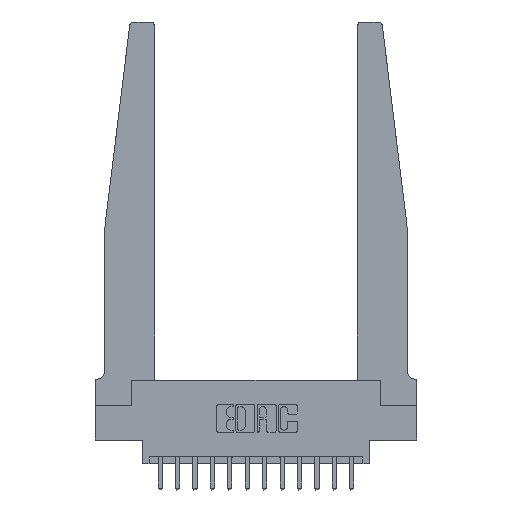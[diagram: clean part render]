
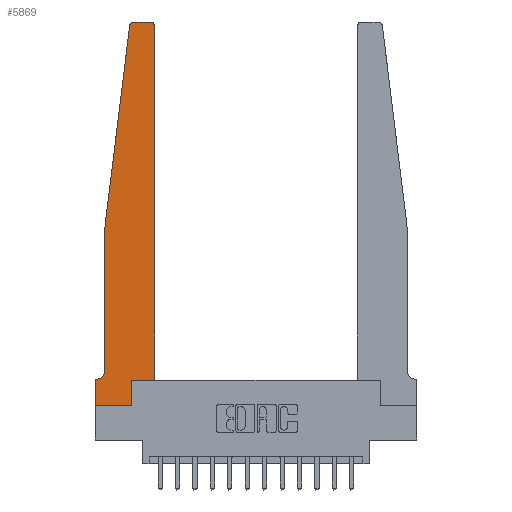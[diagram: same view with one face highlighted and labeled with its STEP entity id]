
A CAD part, top view. The second image highlights one B-rep face of the part: STEP entity #5869.
In plain terms, the highlighted planar face has unit normal (0, 0, 1).
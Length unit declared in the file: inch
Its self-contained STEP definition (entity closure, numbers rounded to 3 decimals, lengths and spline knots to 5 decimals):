
#121 = ORIENTED_EDGE ( 'NONE', *, *, #11067, .T. ) ;
#284 = LINE ( 'NONE', #6180, #6841 ) ;
#321 = EDGE_CURVE ( 'NONE', #11823, #12574, #5708, .T. ) ;
#346 = DIRECTION ( 'NONE',  ( 1., 0., 0. ) ) ;
#353 = CARTESIAN_POINT ( 'NONE',  ( 0.065, 0.2375, 0.37 ) ) ;
#361 = CARTESIAN_POINT ( 'NONE',  ( 0., 0., 0.37 ) ) ;
#403 = CIRCLE ( 'NONE', #14187, 0.05 ) ;
#616 = VECTOR ( 'NONE', #904, 39.37008 ) ;
#721 = CARTESIAN_POINT ( 'NONE',  ( 0.015, 0.1875, 0.37 ) ) ;
#904 = DIRECTION ( 'NONE',  ( -1., 0., 0. ) ) ;
#1146 = DIRECTION ( 'NONE',  ( 0., -1., 0. ) ) ;
#1235 = CARTESIAN_POINT ( 'NONE',  ( 0.065, 1.25, 0.37 ) ) ;
#1589 = VERTEX_POINT ( 'NONE', #13075 ) ;
#1968 = VERTEX_POINT ( 'NONE', #13344 ) ;
#2219 = DIRECTION ( 'NONE',  ( 0., -1., 0. ) ) ;
#2501 = VECTOR ( 'NONE', #2949, 39.37008 ) ;
#2730 = VERTEX_POINT ( 'NONE', #353 ) ;
#2949 = DIRECTION ( 'NONE',  ( 0., 1., 0. ) ) ;
#2978 = LINE ( 'NONE', #1235, #16077 ) ;
#3011 = DIRECTION ( 'NONE',  ( 0., 0., -1. ) ) ;
#3089 = VECTOR ( 'NONE', #10060, 39.37008 ) ;
#3243 = ORIENTED_EDGE ( 'NONE', *, *, #4909, .T. ) ;
#3273 = EDGE_CURVE ( 'NONE', #12574, #16125, #6005, .T. ) ;
#3669 = LINE ( 'NONE', #13989, #616 ) ;
#3678 = CARTESIAN_POINT ( 'NONE',  ( 0.425, 0.18, 0.37 ) ) ;
#3949 = CARTESIAN_POINT ( 'NONE',  ( 0.2605, 0.18, 0.37 ) ) ;
#4288 = CARTESIAN_POINT ( 'NONE',  ( 0., 0.1875, 0.37 ) ) ;
#4425 = LINE ( 'NONE', #361, #4828 ) ;
#4828 = VECTOR ( 'NONE', #346, 39.37008 ) ;
#4901 = CIRCLE ( 'NONE', #8068, 0.03 ) ;
#4909 = EDGE_CURVE ( 'NONE', #10170, #2730, #2978, .T. ) ;
#4979 = CARTESIAN_POINT ( 'NONE',  ( 0.2605, 0.18, 0.37 ) ) ;
#5010 = EDGE_CURVE ( 'NONE', #1589, #12169, #4425, .T. ) ;
#5607 = DIRECTION ( 'NONE',  ( -1., 0., 0. ) ) ;
#5708 = LINE ( 'NONE', #9961, #8782 ) ;
#5761 = ORIENTED_EDGE ( 'NONE', *, *, #14147, .T. ) ;
#5869 = ADVANCED_FACE ( 'NONE', ( #16039 ), #11038, .T. ) ;
#5929 = CARTESIAN_POINT ( 'NONE',  ( 0.065, 1.25, 0.37 ) ) ;
#6005 = LINE ( 'NONE', #3678, #2501 ) ;
#6180 = CARTESIAN_POINT ( 'NONE',  ( 0., 0., 0.37 ) ) ;
#6351 = DIRECTION ( 'NONE',  ( 0., 0., 1. ) ) ;
#6604 = ORIENTED_EDGE ( 'NONE', *, *, #5010, .T. ) ;
#6641 = DIRECTION ( 'NONE',  ( 0., 0., 1. ) ) ;
#6841 = VECTOR ( 'NONE', #2219, 39.37008 ) ;
#7129 = LINE ( 'NONE', #3949, #13311 ) ;
#7538 = EDGE_CURVE ( 'NONE', #1968, #10170, #10120, .T. ) ;
#8068 = AXIS2_PLACEMENT_3D ( 'NONE', #14211, #6351, #15494 ) ;
#8175 = DIRECTION ( 'NONE',  ( 1., 0., 0. ) ) ;
#8308 = CARTESIAN_POINT ( 'NONE',  ( 0.2605, 0., 0.37 ) ) ;
#8378 = ORIENTED_EDGE ( 'NONE', *, *, #9144, .T. ) ;
#8379 = VERTEX_POINT ( 'NONE', #721 ) ;
#8782 = VECTOR ( 'NONE', #8175, 39.37008 ) ;
#8877 = VECTOR ( 'NONE', #5607, 39.37008 ) ;
#9144 = EDGE_CURVE ( 'NONE', #16125, #13365, #4901, .T. ) ;
#9321 = ORIENTED_EDGE ( 'NONE', *, *, #11057, .T. ) ;
#9396 = CARTESIAN_POINT ( 'NONE',  ( 0.425, 0.18, 0.37 ) ) ;
#9822 = CIRCLE ( 'NONE', #14333, 0.03 ) ;
#9961 = CARTESIAN_POINT ( 'NONE',  ( 0.425, 0.18, 0.37 ) ) ;
#10060 = DIRECTION ( 'NONE',  ( -0.122, -0.992, 0. ) ) ;
#10120 = LINE ( 'NONE', #10248, #3089 ) ;
#10170 = VERTEX_POINT ( 'NONE', #5929 ) ;
#10248 = CARTESIAN_POINT ( 'NONE',  ( 0.065, 1.25, 0.37 ) ) ;
#10738 = ORIENTED_EDGE ( 'NONE', *, *, #7538, .T. ) ;
#10868 = CARTESIAN_POINT ( 'NONE',  ( 0.25, 2.75, 0.37 ) ) ;
#10901 = DIRECTION ( 'NONE',  ( 1., 0., 0. ) ) ;
#10922 = DIRECTION ( 'NONE',  ( 0., 0., 1. ) ) ;
#10949 = CARTESIAN_POINT ( 'NONE',  ( 0.015, 0.2375, 0.37 ) ) ;
#11038 = PLANE ( 'NONE',  #15663 ) ;
#11057 = EDGE_CURVE ( 'NONE', #12169, #11823, #7129, .T. ) ;
#11067 = EDGE_CURVE ( 'NONE', #11456, #1968, #9822, .T. ) ;
#11361 = CARTESIAN_POINT ( 'NONE',  ( 0., 0.1875, 0.37 ) ) ;
#11456 = VERTEX_POINT ( 'NONE', #13452 ) ;
#11596 = LINE ( 'NONE', #10868, #8877 ) ;
#11693 = ORIENTED_EDGE ( 'NONE', *, *, #321, .T. ) ;
#11766 = EDGE_CURVE ( 'NONE', #12108, #1589, #284, .T. ) ;
#11823 = VERTEX_POINT ( 'NONE', #4979 ) ;
#11832 = ORIENTED_EDGE ( 'NONE', *, *, #3273, .T. ) ;
#12108 = VERTEX_POINT ( 'NONE', #4288 ) ;
#12169 = VERTEX_POINT ( 'NONE', #8308 ) ;
#12275 = DIRECTION ( 'NONE',  ( -1., 0., 0. ) ) ;
#12574 = VERTEX_POINT ( 'NONE', #9396 ) ;
#12660 = EDGE_CURVE ( 'NONE', #13365, #11456, #11596, .T. ) ;
#13075 = CARTESIAN_POINT ( 'NONE',  ( 0., 0., 0.37 ) ) ;
#13311 = VECTOR ( 'NONE', #14435, 39.37008 ) ;
#13319 = ORIENTED_EDGE ( 'NONE', *, *, #13888, .T. ) ;
#13344 = CARTESIAN_POINT ( 'NONE',  ( 0.24675, 2.72367, 0.37 ) ) ;
#13365 = VERTEX_POINT ( 'NONE', #16134 ) ;
#13452 = CARTESIAN_POINT ( 'NONE',  ( 0.27653, 2.75, 0.37 ) ) ;
#13888 = EDGE_CURVE ( 'NONE', #2730, #8379, #403, .T. ) ;
#13989 = CARTESIAN_POINT ( 'NONE',  ( 0.065, 0.1875, 0.37 ) ) ;
#14147 = EDGE_CURVE ( 'NONE', #8379, #12108, #3669, .T. ) ;
#14187 = AXIS2_PLACEMENT_3D ( 'NONE', #10949, #3011, #12275 ) ;
#14211 = CARTESIAN_POINT ( 'NONE',  ( 0.395, 2.72, 0.37 ) ) ;
#14333 = AXIS2_PLACEMENT_3D ( 'NONE', #14493, #6641, #15769 ) ;
#14435 = DIRECTION ( 'NONE',  ( 0., 1., 0. ) ) ;
#14493 = CARTESIAN_POINT ( 'NONE',  ( 0.27653, 2.72, 0.37 ) ) ;
#14600 = EDGE_LOOP ( 'NONE', ( #16061, #121, #10738, #3243, #13319, #5761, #15089, #6604, #9321, #11693, #11832, #8378 ) ) ;
#15089 = ORIENTED_EDGE ( 'NONE', *, *, #11766, .T. ) ;
#15494 = DIRECTION ( 'NONE',  ( 1., 0., 0. ) ) ;
#15663 = AXIS2_PLACEMENT_3D ( 'NONE', #11361, #10922, #10901 ) ;
#15769 = DIRECTION ( 'NONE',  ( 1., 0., 0. ) ) ;
#16039 = FACE_OUTER_BOUND ( 'NONE', #14600, .T. ) ;
#16061 = ORIENTED_EDGE ( 'NONE', *, *, #12660, .T. ) ;
#16077 = VECTOR ( 'NONE', #1146, 39.37008 ) ;
#16125 = VERTEX_POINT ( 'NONE', #16221 ) ;
#16134 = CARTESIAN_POINT ( 'NONE',  ( 0.395, 2.75, 0.37 ) ) ;
#16221 = CARTESIAN_POINT ( 'NONE',  ( 0.425, 2.72, 0.37 ) ) ;
